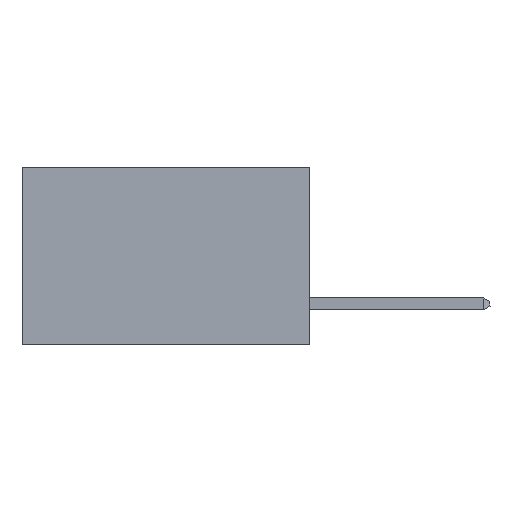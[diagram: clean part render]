
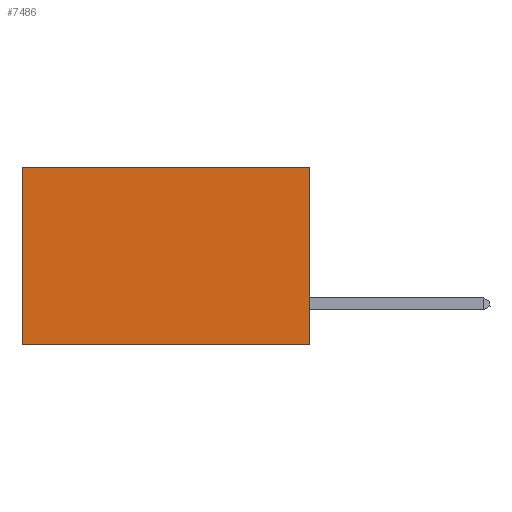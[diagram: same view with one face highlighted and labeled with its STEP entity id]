
A CAD part, left-side view. The second image highlights one B-rep face of the part: STEP entity #7486.
In plain terms, the highlighted planar face has unit normal (-1, 0, 0).
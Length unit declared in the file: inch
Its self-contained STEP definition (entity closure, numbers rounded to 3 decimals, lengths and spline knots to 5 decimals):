
#682 = CARTESIAN_POINT ( 'NONE',  ( 0.2875, 0., 0. ) ) ;
#2044 = DIRECTION ( 'NONE',  ( 0., 1., 0. ) ) ;
#2963 = DIRECTION ( 'NONE',  ( 0., 0., -1. ) ) ;
#3420 = VECTOR ( 'NONE', #2044, 39.37008 ) ;
#4996 = VERTEX_POINT ( 'NONE', #5600 ) ;
#5522 = AXIS2_PLACEMENT_3D ( 'NONE', #682, #16171, #2963 ) ;
#5600 = CARTESIAN_POINT ( 'NONE',  ( 0.2875, 0.6, -0.37 ) ) ;
#6581 = VERTEX_POINT ( 'NONE', #8806 ) ;
#6631 = ORIENTED_EDGE ( 'NONE', *, *, #13152, .F. ) ;
#7028 = EDGE_CURVE ( 'NONE', #7519, #9541, #11960, .T. ) ;
#7486 = ADVANCED_FACE ( 'NONE', ( #16316 ), #11840, .F. ) ;
#7519 = VERTEX_POINT ( 'NONE', #9612 ) ;
#7662 = ORIENTED_EDGE ( 'NONE', *, *, #7028, .F. ) ;
#8099 = DIRECTION ( 'NONE',  ( 0., 0., -1. ) ) ;
#8806 = CARTESIAN_POINT ( 'NONE',  ( 0.2875, 0.6, 0. ) ) ;
#9541 = VERTEX_POINT ( 'NONE', #25987 ) ;
#9569 = CARTESIAN_POINT ( 'NONE',  ( 0.2875, 0., 0. ) ) ;
#9612 = CARTESIAN_POINT ( 'NONE',  ( 0.2875, 0., 0. ) ) ;
#11840 = PLANE ( 'NONE',  #5522 ) ;
#11938 = VECTOR ( 'NONE', #19202, 39.37008 ) ;
#11960 = LINE ( 'NONE', #21094, #22087 ) ;
#12290 = ORIENTED_EDGE ( 'NONE', *, *, #13386, .T. ) ;
#12623 = LINE ( 'NONE', #27709, #11938 ) ;
#13152 = EDGE_CURVE ( 'NONE', #9541, #4996, #20216, .T. ) ;
#13386 = EDGE_CURVE ( 'NONE', #7519, #6581, #14140, .T. ) ;
#14140 = LINE ( 'NONE', #9569, #25512 ) ;
#15000 = EDGE_LOOP ( 'NONE', ( #18550, #6631, #7662, #12290 ) ) ;
#16171 = DIRECTION ( 'NONE',  ( 1., 0., 0. ) ) ;
#16316 = FACE_OUTER_BOUND ( 'NONE', #15000, .T. ) ;
#16592 = EDGE_CURVE ( 'NONE', #6581, #4996, #12623, .T. ) ;
#18550 = ORIENTED_EDGE ( 'NONE', *, *, #16592, .T. ) ;
#19202 = DIRECTION ( 'NONE',  ( 0., 0., -1. ) ) ;
#20216 = LINE ( 'NONE', #21809, #3420 ) ;
#21094 = CARTESIAN_POINT ( 'NONE',  ( 0.2875, 0., 0. ) ) ;
#21809 = CARTESIAN_POINT ( 'NONE',  ( 0.2875, 0., -0.37 ) ) ;
#22087 = VECTOR ( 'NONE', #8099, 39.37008 ) ;
#24635 = DIRECTION ( 'NONE',  ( 0., 1., 0. ) ) ;
#25512 = VECTOR ( 'NONE', #24635, 39.37008 ) ;
#25987 = CARTESIAN_POINT ( 'NONE',  ( 0.2875, 0., -0.37 ) ) ;
#27709 = CARTESIAN_POINT ( 'NONE',  ( 0.2875, 0.6, 0. ) ) ;
